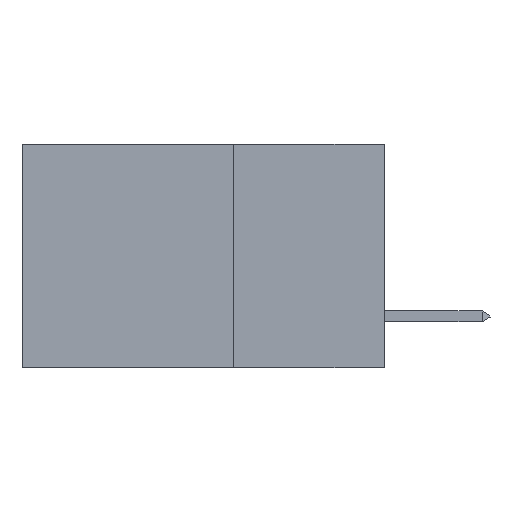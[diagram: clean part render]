
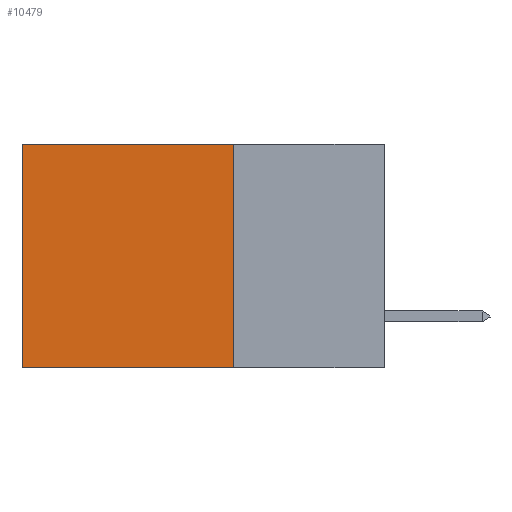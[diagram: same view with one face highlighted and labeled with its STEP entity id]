
A CAD part, left-side view. The second image highlights one B-rep face of the part: STEP entity #10479.
In plain terms, the highlighted planar face has unit normal (-1, 0, 0).
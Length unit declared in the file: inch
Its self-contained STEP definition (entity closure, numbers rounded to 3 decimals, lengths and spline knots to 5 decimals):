
#659 = DIRECTION ( 'NONE',  ( 0., 0., -1. ) ) ;
#859 = LINE ( 'NONE', #17929, #8475 ) ;
#1574 = VERTEX_POINT ( 'NONE', #9542 ) ;
#1991 = PLANE ( 'NONE',  #21306 ) ;
#2403 = CARTESIAN_POINT ( 'NONE',  ( 0.2875, 0.6, 0. ) ) ;
#3574 = EDGE_CURVE ( 'NONE', #15134, #25699, #859, .T. ) ;
#4838 = CARTESIAN_POINT ( 'NONE',  ( 0.2875, 0.6, 0. ) ) ;
#5804 = CARTESIAN_POINT ( 'NONE',  ( 0.2875, 0.25, 0. ) ) ;
#6031 = DIRECTION ( 'NONE',  ( 0., 1., 0. ) ) ;
#6749 = CARTESIAN_POINT ( 'NONE',  ( 0.2875, 0.25, 0. ) ) ;
#8403 = EDGE_CURVE ( 'NONE', #25699, #21483, #13863, .T. ) ;
#8475 = VECTOR ( 'NONE', #6031, 39.37008 ) ;
#9542 = CARTESIAN_POINT ( 'NONE',  ( 0.2875, 0.25, -0.37 ) ) ;
#9892 = DIRECTION ( 'NONE',  ( 1., 0., 0. ) ) ;
#10055 = EDGE_CURVE ( 'NONE', #15134, #1574, #13456, .T. ) ;
#10479 = ADVANCED_FACE ( 'NONE', ( #17248 ), #1991, .F. ) ;
#10665 = DIRECTION ( 'NONE',  ( 0., 0., -1. ) ) ;
#12289 = ORIENTED_EDGE ( 'NONE', *, *, #18307, .F. ) ;
#13025 = VECTOR ( 'NONE', #19585, 39.37008 ) ;
#13456 = LINE ( 'NONE', #18882, #17535 ) ;
#13863 = LINE ( 'NONE', #2403, #20503 ) ;
#14111 = ORIENTED_EDGE ( 'NONE', *, *, #8403, .T. ) ;
#14217 = DIRECTION ( 'NONE',  ( 0., 0., -1. ) ) ;
#15134 = VERTEX_POINT ( 'NONE', #6749 ) ;
#15267 = EDGE_LOOP ( 'NONE', ( #14111, #12289, #23058, #23900 ) ) ;
#15529 = LINE ( 'NONE', #19762, #13025 ) ;
#17248 = FACE_OUTER_BOUND ( 'NONE', #15267, .T. ) ;
#17535 = VECTOR ( 'NONE', #659, 39.37008 ) ;
#17929 = CARTESIAN_POINT ( 'NONE',  ( 0.2875, 0.25, 0. ) ) ;
#18258 = CARTESIAN_POINT ( 'NONE',  ( 0.2875, 0.6, -0.37 ) ) ;
#18307 = EDGE_CURVE ( 'NONE', #1574, #21483, #15529, .T. ) ;
#18882 = CARTESIAN_POINT ( 'NONE',  ( 0.2875, 0.25, 0. ) ) ;
#19585 = DIRECTION ( 'NONE',  ( 0., 1., 0. ) ) ;
#19762 = CARTESIAN_POINT ( 'NONE',  ( 0.2875, 0.25, -0.37 ) ) ;
#20503 = VECTOR ( 'NONE', #10665, 39.37008 ) ;
#21306 = AXIS2_PLACEMENT_3D ( 'NONE', #5804, #9892, #14217 ) ;
#21483 = VERTEX_POINT ( 'NONE', #18258 ) ;
#23058 = ORIENTED_EDGE ( 'NONE', *, *, #10055, .F. ) ;
#23900 = ORIENTED_EDGE ( 'NONE', *, *, #3574, .T. ) ;
#25699 = VERTEX_POINT ( 'NONE', #4838 ) ;
